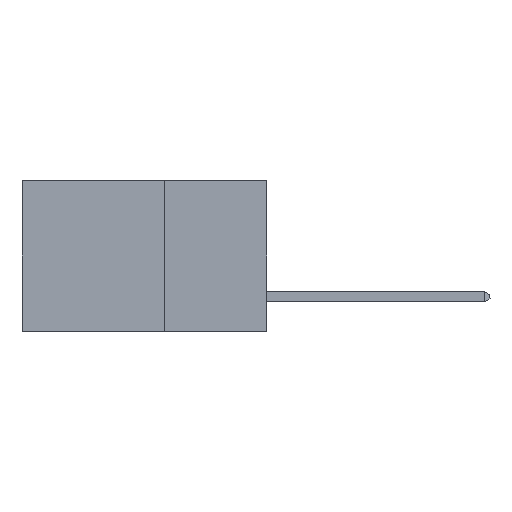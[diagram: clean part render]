
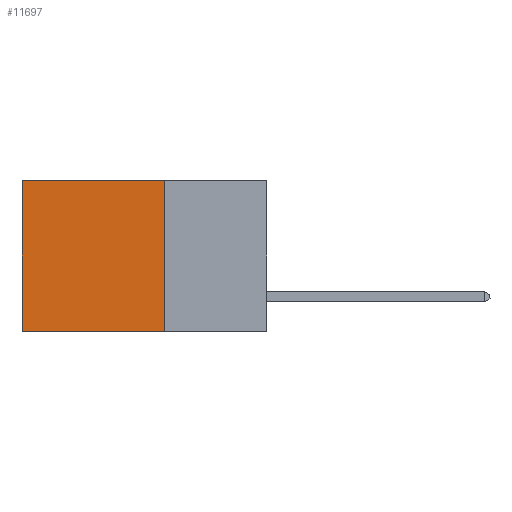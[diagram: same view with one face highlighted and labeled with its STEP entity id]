
A CAD part, left-side view. The second image highlights one B-rep face of the part: STEP entity #11697.
In plain terms, the highlighted planar face has unit normal (-1, 0, 0).
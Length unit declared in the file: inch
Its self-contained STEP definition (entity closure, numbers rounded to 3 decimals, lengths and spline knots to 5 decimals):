
#461 = AXIS2_PLACEMENT_3D ( 'NONE', #10059, #2470, #6341 ) ;
#479 = VECTOR ( 'NONE', #9614, 39.37008 ) ;
#594 = DIRECTION ( 'NONE',  ( 0., 1., 0. ) ) ;
#931 = EDGE_LOOP ( 'NONE', ( #9438, #11524, #6735, #11671 ) ) ;
#1377 = CARTESIAN_POINT ( 'NONE',  ( 0.2875, 0.25, -0.37 ) ) ;
#1835 = VECTOR ( 'NONE', #4396, 39.37008 ) ;
#2430 = FACE_OUTER_BOUND ( 'NONE', #931, .T. ) ;
#2470 = DIRECTION ( 'NONE',  ( 1., 0., 0. ) ) ;
#2773 = LINE ( 'NONE', #1377, #10046 ) ;
#2804 = EDGE_CURVE ( 'NONE', #4019, #3278, #2773, .T. ) ;
#2985 = LINE ( 'NONE', #8671, #479 ) ;
#3278 = VERTEX_POINT ( 'NONE', #6436 ) ;
#3895 = VERTEX_POINT ( 'NONE', #7751 ) ;
#4019 = VERTEX_POINT ( 'NONE', #8453 ) ;
#4396 = DIRECTION ( 'NONE',  ( 0., 1., 0. ) ) ;
#4582 = VERTEX_POINT ( 'NONE', #4889 ) ;
#4889 = CARTESIAN_POINT ( 'NONE',  ( 0.2875, 0.25, 0. ) ) ;
#5405 = PLANE ( 'NONE',  #461 ) ;
#5571 = EDGE_CURVE ( 'NONE', #4582, #3895, #9398, .T. ) ;
#6341 = DIRECTION ( 'NONE',  ( 0., 0., -1. ) ) ;
#6436 = CARTESIAN_POINT ( 'NONE',  ( 0.2875, 0.6, -0.37 ) ) ;
#6735 = ORIENTED_EDGE ( 'NONE', *, *, #11042, .F. ) ;
#7258 = CARTESIAN_POINT ( 'NONE',  ( 0.2875, 0.25, 0. ) ) ;
#7290 = EDGE_CURVE ( 'NONE', #3895, #3278, #2985, .T. ) ;
#7751 = CARTESIAN_POINT ( 'NONE',  ( 0.2875, 0.6, 0. ) ) ;
#8131 = CARTESIAN_POINT ( 'NONE',  ( 0.2875, 0.25, 0. ) ) ;
#8453 = CARTESIAN_POINT ( 'NONE',  ( 0.2875, 0.25, -0.37 ) ) ;
#8671 = CARTESIAN_POINT ( 'NONE',  ( 0.2875, 0.6, 0. ) ) ;
#9275 = VECTOR ( 'NONE', #10072, 39.37008 ) ;
#9398 = LINE ( 'NONE', #8131, #1835 ) ;
#9438 = ORIENTED_EDGE ( 'NONE', *, *, #7290, .T. ) ;
#9614 = DIRECTION ( 'NONE',  ( 0., 0., -1. ) ) ;
#10046 = VECTOR ( 'NONE', #594, 39.37008 ) ;
#10059 = CARTESIAN_POINT ( 'NONE',  ( 0.2875, 0.25, 0. ) ) ;
#10072 = DIRECTION ( 'NONE',  ( 0., 0., -1. ) ) ;
#11042 = EDGE_CURVE ( 'NONE', #4582, #4019, #11763, .T. ) ;
#11524 = ORIENTED_EDGE ( 'NONE', *, *, #2804, .F. ) ;
#11671 = ORIENTED_EDGE ( 'NONE', *, *, #5571, .T. ) ;
#11697 = ADVANCED_FACE ( 'NONE', ( #2430 ), #5405, .F. ) ;
#11763 = LINE ( 'NONE', #7258, #9275 ) ;
